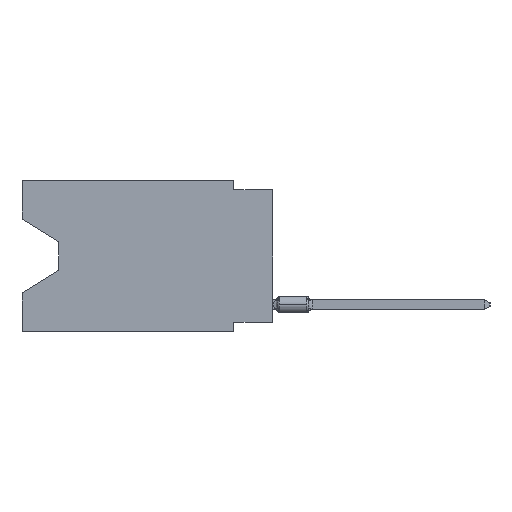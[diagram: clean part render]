
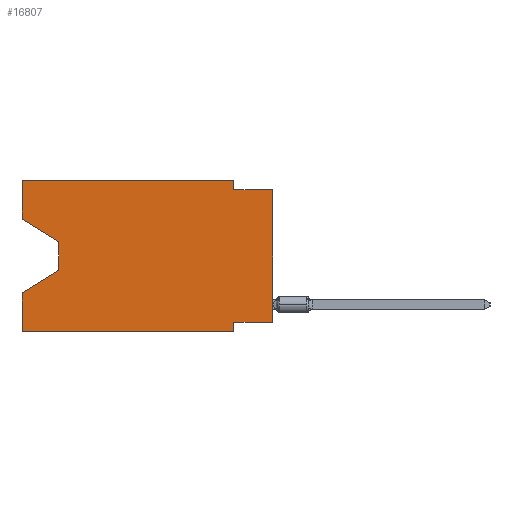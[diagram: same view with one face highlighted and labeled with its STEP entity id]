
A CAD part, left-side view. The second image highlights one B-rep face of the part: STEP entity #16807.
In plain terms, the highlighted planar face has unit normal (-1, 0, 0).
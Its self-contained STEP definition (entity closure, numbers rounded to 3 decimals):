
#113 = VERTEX_POINT ( 'NONE', #24143 ) ;
#325 = LINE ( 'NONE', #24645, #2174 ) ;
#409 = VERTEX_POINT ( 'NONE', #14361 ) ;
#413 = DIRECTION ( 'NONE',  ( 0., -1., 0. ) ) ;
#466 = EDGE_CURVE ( 'NONE', #3988, #7822, #16822, .T. ) ;
#1002 = ORIENTED_EDGE ( 'NONE', *, *, #466, .F. ) ;
#1212 = VECTOR ( 'NONE', #27781, 1000. ) ;
#1279 = CARTESIAN_POINT ( 'NONE',  ( 0., 16.383, 0. ) ) ;
#1312 = CARTESIAN_POINT ( 'NONE',  ( 0., 16.383, 0. ) ) ;
#1558 = VERTEX_POINT ( 'NONE', #9236 ) ;
#1655 = DIRECTION ( 'NONE',  ( 0., 0.855, -0.519 ) ) ;
#1892 = VERTEX_POINT ( 'NONE', #16733 ) ;
#2174 = VECTOR ( 'NONE', #14715, 1000. ) ;
#2217 = EDGE_CURVE ( 'NONE', #25856, #409, #22506, .T. ) ;
#2813 = DIRECTION ( 'NONE',  ( 0., -1., 0. ) ) ;
#3988 = VERTEX_POINT ( 'NONE', #30245 ) ;
#4146 = ORIENTED_EDGE ( 'NONE', *, *, #14470, .F. ) ;
#4184 = VERTEX_POINT ( 'NONE', #7147 ) ;
#4909 = VECTOR ( 'NONE', #29644, 1000. ) ;
#4918 = ORIENTED_EDGE ( 'NONE', *, *, #6170, .F. ) ;
#5102 = DIRECTION ( 'NONE',  ( 0., -0.855, -0.519 ) ) ;
#5152 = CARTESIAN_POINT ( 'NONE',  ( 0., 16.383, -9.906 ) ) ;
#5266 = EDGE_CURVE ( 'NONE', #12007, #113, #325, .T. ) ;
#5853 = DIRECTION ( 'NONE',  ( 0., 0., -1. ) ) ;
#6170 = EDGE_CURVE ( 'NONE', #409, #4184, #22684, .T. ) ;
#6416 = EDGE_CURVE ( 'NONE', #4184, #3988, #14720, .T. ) ;
#6820 = CARTESIAN_POINT ( 'NONE',  ( 0., 0., -9.271 ) ) ;
#7147 = CARTESIAN_POINT ( 'NONE',  ( 0., 2.54, 0. ) ) ;
#7822 = VERTEX_POINT ( 'NONE', #11231 ) ;
#8426 = ORIENTED_EDGE ( 'NONE', *, *, #19278, .F. ) ;
#8886 = VECTOR ( 'NONE', #10710, 1000. ) ;
#9112 = ORIENTED_EDGE ( 'NONE', *, *, #30592, .T. ) ;
#9193 = VECTOR ( 'NONE', #14510, 1000. ) ;
#9236 = CARTESIAN_POINT ( 'NONE',  ( 0., 2.54, -9.906 ) ) ;
#9375 = CARTESIAN_POINT ( 'NONE',  ( 0., 2.54, -9.271 ) ) ;
#9770 = LINE ( 'NONE', #5152, #24197 ) ;
#10392 = VERTEX_POINT ( 'NONE', #9375 ) ;
#10710 = DIRECTION ( 'NONE',  ( 0., 0., 1. ) ) ;
#11231 = CARTESIAN_POINT ( 'NONE',  ( 0., 0., -0.635 ) ) ;
#11303 = VECTOR ( 'NONE', #12892, 1000. ) ;
#11349 = CARTESIAN_POINT ( 'NONE',  ( 0., 0., 0. ) ) ;
#11426 = ORIENTED_EDGE ( 'NONE', *, *, #21566, .F. ) ;
#11875 = VERTEX_POINT ( 'NONE', #30241 ) ;
#12007 = VERTEX_POINT ( 'NONE', #26816 ) ;
#12892 = DIRECTION ( 'NONE',  ( 0., 0., -1. ) ) ;
#13101 = VECTOR ( 'NONE', #5102, 1000. ) ;
#14361 = CARTESIAN_POINT ( 'NONE',  ( 0., 16.383, 0. ) ) ;
#14470 = EDGE_CURVE ( 'NONE', #10392, #1558, #27072, .T. ) ;
#14509 = EDGE_LOOP ( 'NONE', ( #9112, #15624, #26737, #8426, #24119, #4146, #11426, #24247, #1002, #29927, #4918, #20790 ) ) ;
#14510 = DIRECTION ( 'NONE',  ( 0., 1., 0. ) ) ;
#14515 = CARTESIAN_POINT ( 'NONE',  ( 0., 0., -0.635 ) ) ;
#14715 = DIRECTION ( 'NONE',  ( 0., 0., -1. ) ) ;
#14720 = LINE ( 'NONE', #24178, #11303 ) ;
#15624 = ORIENTED_EDGE ( 'NONE', *, *, #5266, .T. ) ;
#16658 = LINE ( 'NONE', #17130, #9193 ) ;
#16733 = CARTESIAN_POINT ( 'NONE',  ( 0., 16.383, -9.906 ) ) ;
#16807 = ADVANCED_FACE ( 'NONE', ( #27560 ), #22621, .F. ) ;
#16822 = LINE ( 'NONE', #14515, #25362 ) ;
#17130 = CARTESIAN_POINT ( 'NONE',  ( 0., 0., -9.271 ) ) ;
#17143 = CARTESIAN_POINT ( 'NONE',  ( 0., 2.54, -9.906 ) ) ;
#18369 = LINE ( 'NONE', #25497, #23401 ) ;
#18929 = LINE ( 'NONE', #11349, #1212 ) ;
#19278 = EDGE_CURVE ( 'NONE', #1892, #11875, #20623, .T. ) ;
#19523 = VERTEX_POINT ( 'NONE', #6820 ) ;
#19775 = CARTESIAN_POINT ( 'NONE',  ( 0., 16.383, -2.546 ) ) ;
#20623 = LINE ( 'NONE', #24985, #21621 ) ;
#20790 = ORIENTED_EDGE ( 'NONE', *, *, #2217, .F. ) ;
#21337 = VECTOR ( 'NONE', #5853, 1000. ) ;
#21366 = LINE ( 'NONE', #19775, #13101 ) ;
#21566 = EDGE_CURVE ( 'NONE', #19523, #10392, #16658, .T. ) ;
#21621 = VECTOR ( 'NONE', #29606, 1000. ) ;
#22506 = LINE ( 'NONE', #1279, #8886 ) ;
#22621 = PLANE ( 'NONE',  #24939 ) ;
#22684 = LINE ( 'NONE', #1312, #4909 ) ;
#23401 = VECTOR ( 'NONE', #1655, 1000. ) ;
#24119 = ORIENTED_EDGE ( 'NONE', *, *, #24251, .T. ) ;
#24143 = CARTESIAN_POINT ( 'NONE',  ( 0., 13.97, -5.893 ) ) ;
#24178 = CARTESIAN_POINT ( 'NONE',  ( 0., 2.54, 0. ) ) ;
#24197 = VECTOR ( 'NONE', #2813, 1000. ) ;
#24247 = ORIENTED_EDGE ( 'NONE', *, *, #30073, .T. ) ;
#24251 = EDGE_CURVE ( 'NONE', #1892, #1558, #9770, .T. ) ;
#24645 = CARTESIAN_POINT ( 'NONE',  ( 0., 13.97, -4.013 ) ) ;
#24939 = AXIS2_PLACEMENT_3D ( 'NONE', #27260, #25250, #24953 ) ;
#24953 = DIRECTION ( 'NONE',  ( 0., 0., -1. ) ) ;
#24985 = CARTESIAN_POINT ( 'NONE',  ( 0., 16.383, 0. ) ) ;
#25250 = DIRECTION ( 'NONE',  ( 1., 0., 0. ) ) ;
#25362 = VECTOR ( 'NONE', #413, 1000. ) ;
#25497 = CARTESIAN_POINT ( 'NONE',  ( 0., 13.97, -5.893 ) ) ;
#25856 = VERTEX_POINT ( 'NONE', #27716 ) ;
#26737 = ORIENTED_EDGE ( 'NONE', *, *, #29084, .T. ) ;
#26816 = CARTESIAN_POINT ( 'NONE',  ( 0., 13.97, -4.013 ) ) ;
#27072 = LINE ( 'NONE', #17143, #21337 ) ;
#27260 = CARTESIAN_POINT ( 'NONE',  ( 0., 16.383, 0. ) ) ;
#27560 = FACE_OUTER_BOUND ( 'NONE', #14509, .T. ) ;
#27716 = CARTESIAN_POINT ( 'NONE',  ( 0., 16.383, -2.546 ) ) ;
#27781 = DIRECTION ( 'NONE',  ( 0., 0., 1. ) ) ;
#29084 = EDGE_CURVE ( 'NONE', #113, #11875, #18369, .T. ) ;
#29606 = DIRECTION ( 'NONE',  ( 0., 0., 1. ) ) ;
#29644 = DIRECTION ( 'NONE',  ( 0., -1., 0. ) ) ;
#29927 = ORIENTED_EDGE ( 'NONE', *, *, #6416, .F. ) ;
#30073 = EDGE_CURVE ( 'NONE', #19523, #7822, #18929, .T. ) ;
#30241 = CARTESIAN_POINT ( 'NONE',  ( 0., 16.383, -7.36 ) ) ;
#30245 = CARTESIAN_POINT ( 'NONE',  ( 0., 2.54, -0.635 ) ) ;
#30592 = EDGE_CURVE ( 'NONE', #25856, #12007, #21366, .T. ) ;
